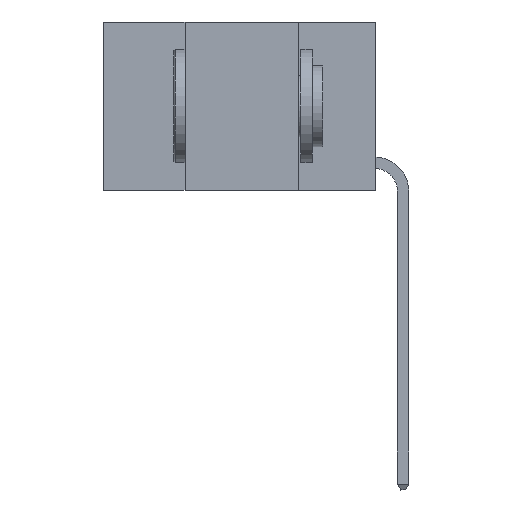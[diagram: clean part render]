
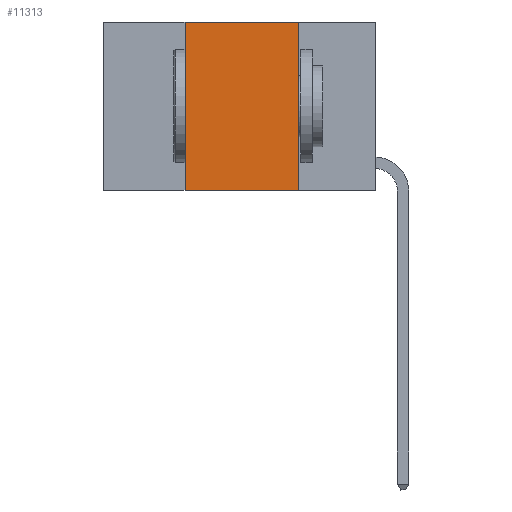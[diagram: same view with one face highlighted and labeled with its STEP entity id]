
A CAD part, left-side view. The second image highlights one B-rep face of the part: STEP entity #11313.
In plain terms, the highlighted planar face has unit normal (-1, 0, 0).
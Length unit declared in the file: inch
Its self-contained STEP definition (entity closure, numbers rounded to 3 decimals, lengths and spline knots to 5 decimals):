
#655 = EDGE_CURVE ( 'NONE', #10661, #12423, #734, .T. ) ;
#734 = LINE ( 'NONE', #3952, #8967 ) ;
#1542 = ORIENTED_EDGE ( 'NONE', *, *, #655, .F. ) ;
#2043 = EDGE_CURVE ( 'NONE', #12199, #9227, #7189, .T. ) ;
#2132 = ORIENTED_EDGE ( 'NONE', *, *, #2043, .F. ) ;
#2446 = CARTESIAN_POINT ( 'NONE',  ( 0., 0.17, 0. ) ) ;
#2718 = VECTOR ( 'NONE', #12271, 39.37008 ) ;
#3952 = CARTESIAN_POINT ( 'NONE',  ( 0., 0.42, 0. ) ) ;
#4421 = VECTOR ( 'NONE', #5875, 39.37008 ) ;
#5315 = CARTESIAN_POINT ( 'NONE',  ( 0., 0.6, 0. ) ) ;
#5875 = DIRECTION ( 'NONE',  ( 0., 0., -1. ) ) ;
#6271 = CARTESIAN_POINT ( 'NONE',  ( 0., 0.17, -0.37 ) ) ;
#6308 = CARTESIAN_POINT ( 'NONE',  ( 0., 0.42, 0. ) ) ;
#6392 = DIRECTION ( 'NONE',  ( 0., 0., -1. ) ) ;
#6709 = CARTESIAN_POINT ( 'NONE',  ( 0., 0.6, -0.37 ) ) ;
#6975 = DIRECTION ( 'NONE',  ( 0., 0., 1. ) ) ;
#7189 = LINE ( 'NONE', #2446, #4421 ) ;
#7192 = AXIS2_PLACEMENT_3D ( 'NONE', #5315, #12453, #6392 ) ;
#7350 = PLANE ( 'NONE',  #7192 ) ;
#7488 = VECTOR ( 'NONE', #9789, 39.37008 ) ;
#7853 = EDGE_CURVE ( 'NONE', #10661, #9227, #10219, .T. ) ;
#8088 = CARTESIAN_POINT ( 'NONE',  ( 0., 0.42, -0.37 ) ) ;
#8967 = VECTOR ( 'NONE', #6975, 39.37008 ) ;
#9227 = VERTEX_POINT ( 'NONE', #6271 ) ;
#9497 = FACE_OUTER_BOUND ( 'NONE', #9715, .T. ) ;
#9715 = EDGE_LOOP ( 'NONE', ( #2132, #10370, #1542, #13133 ) ) ;
#9789 = DIRECTION ( 'NONE',  ( 0., -1., 0. ) ) ;
#10219 = LINE ( 'NONE', #6709, #7488 ) ;
#10276 = CARTESIAN_POINT ( 'NONE',  ( 0., 0.6, 0. ) ) ;
#10370 = ORIENTED_EDGE ( 'NONE', *, *, #13164, .F. ) ;
#10620 = LINE ( 'NONE', #10276, #2718 ) ;
#10661 = VERTEX_POINT ( 'NONE', #8088 ) ;
#11313 = ADVANCED_FACE ( 'NONE', ( #9497 ), #7350, .F. ) ;
#12040 = CARTESIAN_POINT ( 'NONE',  ( 0., 0.17, 0. ) ) ;
#12199 = VERTEX_POINT ( 'NONE', #12040 ) ;
#12271 = DIRECTION ( 'NONE',  ( 0., -1., 0. ) ) ;
#12423 = VERTEX_POINT ( 'NONE', #6308 ) ;
#12453 = DIRECTION ( 'NONE',  ( 1., 0., 0. ) ) ;
#13133 = ORIENTED_EDGE ( 'NONE', *, *, #7853, .T. ) ;
#13164 = EDGE_CURVE ( 'NONE', #12423, #12199, #10620, .T. ) ;
